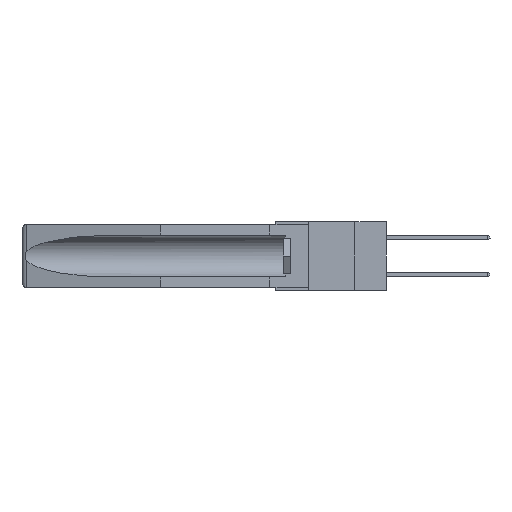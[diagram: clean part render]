
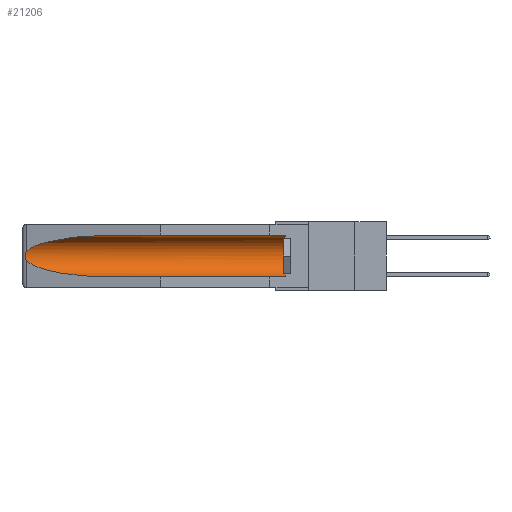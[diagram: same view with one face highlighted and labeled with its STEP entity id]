
A CAD part, left-side view. The second image highlights one B-rep face of the part: STEP entity #21206.
In plain terms, the highlighted cylindrical face has radius 2.857 mm (diameter 5.715 mm), a partial arc.
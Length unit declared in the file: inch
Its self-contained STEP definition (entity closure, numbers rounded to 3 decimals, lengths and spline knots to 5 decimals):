
#100 = CARTESIAN_POINT ( 'NONE',  ( 0.21114, 1.30732, -0.284 ) ) ;
#1146 = CARTESIAN_POINT ( 'NONE',  ( 0.26597, 1.5296, -0.19026 ) ) ;
#1297 = VERTEX_POINT ( 'NONE', #15570 ) ;
#1869 = CARTESIAN_POINT ( 'NONE',  ( 0.26537, 1.52718, -0.19328 ) ) ;
#1942 = CARTESIAN_POINT ( 'NONE',  ( 0.155, 1.07973, -0.284 ) ) ;
#2185 = CARTESIAN_POINT ( 'NONE',  ( 0.155, 1.07973, -0.059 ) ) ;
#2953 = CYLINDRICAL_SURFACE ( 'NONE', #10782, 0.1125 ) ;
#3250 = ORIENTED_EDGE ( 'NONE', *, *, #19216, .T. ) ;
#3319 = CARTESIAN_POINT ( 'NONE',  ( 0.155, -0.30754, -0.1715 ) ) ;
#3646 = DIRECTION ( 'NONE',  ( 0., 1., 0. ) ) ;
#3787 = CARTESIAN_POINT ( 'NONE',  ( 0.2673, 1.5327, -0.16383 ) ) ;
#4139 = VERTEX_POINT ( 'NONE', #20425 ) ;
#5045 = LINE ( 'NONE', #10179, #20158 ) ;
#5527 = EDGE_CURVE ( 'NONE', #18081, #18370, #5045, .T. ) ;
#5608 = CARTESIAN_POINT ( 'NONE',  ( 0.21114, 1.30732, -0.059 ) ) ;
#5619 = CARTESIAN_POINT ( 'NONE',  ( 0.26654, 1.53092, -0.15636 ) ) ;
#5832 = AXIS2_PLACEMENT_3D ( 'NONE', #8442, #11950, #8719 ) ;
#6144 = LINE ( 'NONE', #14553, #17866 ) ;
#6628 = FACE_OUTER_BOUND ( 'NONE', #7625, .T. ) ;
#6963 = EDGE_CURVE ( 'NONE', #13067, #18370, #11127, .T. ) ;
#7625 = EDGE_LOOP ( 'NONE', ( #3250, #9653, #17619, #20986, #14206, #14065 ) ) ;
#7726 = CARTESIAN_POINT ( 'NONE',  ( 0.26537, 1.52718, -0.19328 ) ) ;
#8240 = DIRECTION ( 'NONE',  ( 0., 0., 1. ) ) ;
#8442 = CARTESIAN_POINT ( 'NONE',  ( 0.155, 0.126, -0.1715 ) ) ;
#8719 = DIRECTION ( 'NONE',  ( 0., 0., 1. ) ) ;
#9653 = ORIENTED_EDGE ( 'NONE', *, *, #17570, .T. ) ;
#9864 = CARTESIAN_POINT ( 'NONE',  ( 0.155, 1.07973, -0.284 ) ) ;
#10065 = DIRECTION ( 'NONE',  ( 0., 1., 0. ) ) ;
#10179 = CARTESIAN_POINT ( 'NONE',  ( 0.155, -0.30754, -0.284 ) ) ;
#10714 = VERTEX_POINT ( 'NONE', #11077 ) ;
#10782 = AXIS2_PLACEMENT_3D ( 'NONE', #3319, #10065, #8240 ) ;
#11077 = CARTESIAN_POINT ( 'NONE',  ( 0.26537, 1.52718, -0.14972 ) ) ;
#11127 =( BOUNDED_CURVE ( )  B_SPLINE_CURVE ( 3, ( #1869, #11876, #100, #1942 ),
 .UNSPECIFIED., .F., .T. ) 
 B_SPLINE_CURVE_WITH_KNOTS ( ( 4, 4 ),
 ( 0.1948, 1.5708 ),
 .UNSPECIFIED. ) 
 CURVE ( )  GEOMETRIC_REPRESENTATION_ITEM ( )  RATIONAL_B_SPLINE_CURVE ( ( 1., 0.848, 0.848, 1. ) ) 
 REPRESENTATION_ITEM ( '' )  );
#11541 = CARTESIAN_POINT ( 'NONE',  ( 0.2673, 1.53269, -0.17917 ) ) ;
#11876 = CARTESIAN_POINT ( 'NONE',  ( 0.25451, 1.48313, -0.24835 ) ) ;
#11950 = DIRECTION ( 'NONE',  ( 0., -1., 0. ) ) ;
#12054 = EDGE_CURVE ( 'NONE', #1297, #4139, #6144, .T. ) ;
#12208 = CARTESIAN_POINT ( 'NONE',  ( 0.26537, 1.52718, -0.19328 ) ) ;
#12242 = CARTESIAN_POINT ( 'NONE',  ( 0.25451, 1.48313, -0.09465 ) ) ;
#12740 = CIRCLE ( 'NONE', #5832, 0.1125 ) ;
#13067 = VERTEX_POINT ( 'NONE', #12208 ) ;
#13109 = DIRECTION ( 'NONE',  ( 0., 1., 0. ) ) ;
#13391 = B_SPLINE_CURVE_WITH_KNOTS ( 'NONE', 3,
 ( #21165, #15206, #5619, #3787, #21341, #16160, #11541, #17791, #1146, #7726 ),
 .UNSPECIFIED., .F., .F.,
 ( 4, 2, 2, 2, 4 ),
 ( 0., 0.00029, 0.00058, 0.00087, 0.00117 ),
 .UNSPECIFIED. ) ;
#13707 = CARTESIAN_POINT ( 'NONE',  ( 0.26537, 1.52718, -0.14972 ) ) ;
#14065 = ORIENTED_EDGE ( 'NONE', *, *, #12054, .T. ) ;
#14206 = ORIENTED_EDGE ( 'NONE', *, *, #16742, .T. ) ;
#14553 = CARTESIAN_POINT ( 'NONE',  ( 0.155, -0.30754, -0.059 ) ) ;
#15206 = CARTESIAN_POINT ( 'NONE',  ( 0.26597, 1.52961, -0.15275 ) ) ;
#15291 =( BOUNDED_CURVE ( )  B_SPLINE_CURVE ( 3, ( #2185, #5608, #12242, #13707 ),
 .UNSPECIFIED., .F., .F. ) 
 B_SPLINE_CURVE_WITH_KNOTS ( ( 4, 4 ),
 ( 4.71239, 6.08839 ),
 .UNSPECIFIED. ) 
 CURVE ( )  GEOMETRIC_REPRESENTATION_ITEM ( )  RATIONAL_B_SPLINE_CURVE ( ( 1., 0.848, 0.848, 1. ) ) 
 REPRESENTATION_ITEM ( '' )  );
#15570 = CARTESIAN_POINT ( 'NONE',  ( 0.155, 0.126, -0.059 ) ) ;
#16160 = CARTESIAN_POINT ( 'NONE',  ( 0.2675, 1.53308, -0.17534 ) ) ;
#16742 = EDGE_CURVE ( 'NONE', #18081, #1297, #12740, .T. ) ;
#17570 = EDGE_CURVE ( 'NONE', #10714, #13067, #13391, .T. ) ;
#17619 = ORIENTED_EDGE ( 'NONE', *, *, #6963, .T. ) ;
#17791 = CARTESIAN_POINT ( 'NONE',  ( 0.26655, 1.53094, -0.18657 ) ) ;
#17866 = VECTOR ( 'NONE', #13109, 39.37008 ) ;
#18081 = VERTEX_POINT ( 'NONE', #19084 ) ;
#18370 = VERTEX_POINT ( 'NONE', #9864 ) ;
#19084 = CARTESIAN_POINT ( 'NONE',  ( 0.155, 0.126, -0.284 ) ) ;
#19216 = EDGE_CURVE ( 'NONE', #4139, #10714, #15291, .T. ) ;
#20158 = VECTOR ( 'NONE', #3646, 39.37008 ) ;
#20425 = CARTESIAN_POINT ( 'NONE',  ( 0.155, 1.07973, -0.059 ) ) ;
#20986 = ORIENTED_EDGE ( 'NONE', *, *, #5527, .F. ) ;
#21165 = CARTESIAN_POINT ( 'NONE',  ( 0.26537, 1.52718, -0.14972 ) ) ;
#21206 = ADVANCED_FACE ( 'NONE', ( #6628 ), #2953, .F. ) ;
#21341 = CARTESIAN_POINT ( 'NONE',  ( 0.2675, 1.53308, -0.16763 ) ) ;
